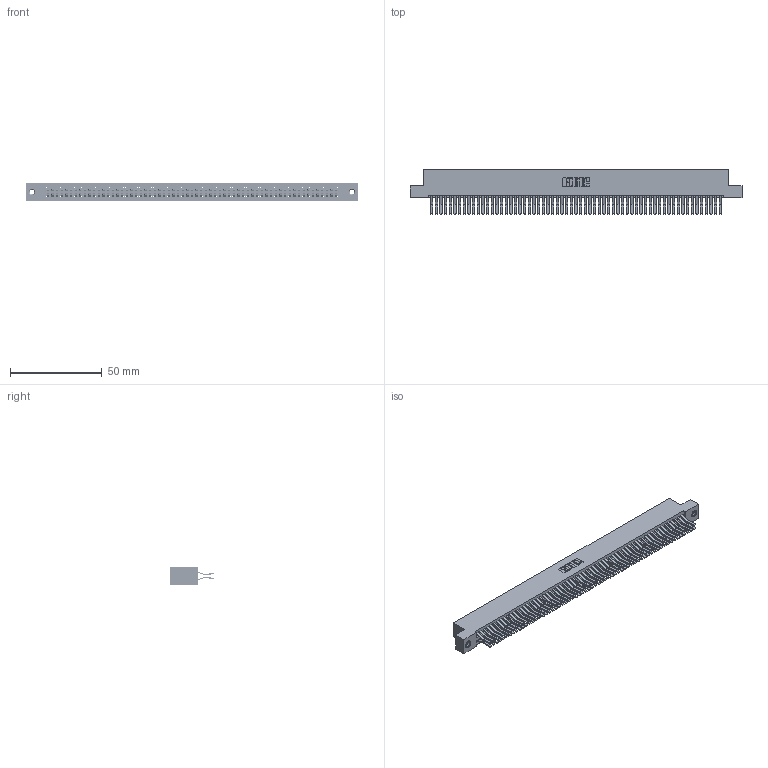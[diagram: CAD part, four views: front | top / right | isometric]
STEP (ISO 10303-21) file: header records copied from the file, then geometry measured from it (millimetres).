
FILE_DESCRIPTION (( 'STEP AP203' ), '1' );
FILE_NAME ('395-126-560-207.STEP', '2019-10-28T17:14:32', ( '' ), ( '' ), 'SwSTEP 2.0', 'SolidWorks 2016', '' );
FILE_SCHEMA (( 'CONFIG_CONTROL_DESIGN' ));
Length unit declared in the file: inch
Products named in the file (4): 345-250-001_345-250-005-103; 395-126-560-207; 345 Part_Flush Mounting Lugs - 0.156 Dia-TI; 345-292-001_560 Tail
Assembly tree (129 placements, depth 2):
  395-126-560-207
    345 Part_Flush Mounting Lugs - 0.156 Dia-TI
    345-292-001_560 Tail  x126
    345-250-001_345-250-005-103  x2
Bounding box: 181.23 x 24.45 x 9.4 mm (x, y, z)
Volume: 18612.1 mm3; surface area: 30070.4 mm2
Topology: 129 solids, 129 shells, 6738 faces, 20007 edges, 13162 vertices
Faces by surface type: plane 4270, cylinder 2452, cone 12, torus 4
Entity records: 47878 total; most frequent: CARTESIAN_POINT 7987, ORIENTED_EDGE 7914, DIRECTION 7047, EDGE_CURVE 3957, VECTOR 3549, LINE 3549, VERTEX_POINT 2632, AXIS2_PLACEMENT_3D 1749
